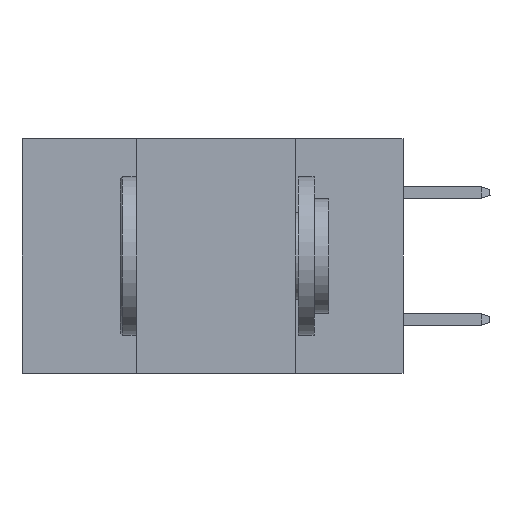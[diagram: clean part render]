
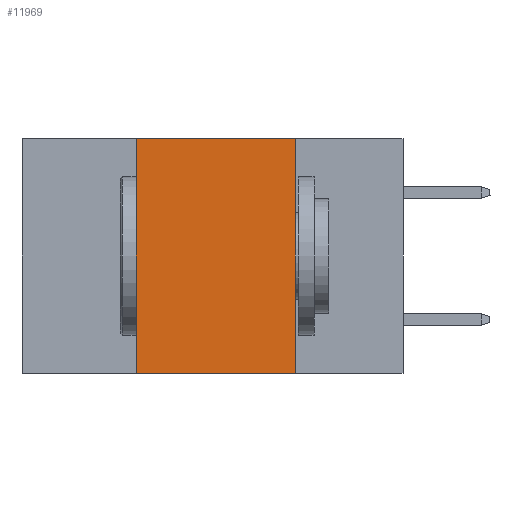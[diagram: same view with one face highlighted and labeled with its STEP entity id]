
A CAD part, left-side view. The second image highlights one B-rep face of the part: STEP entity #11969.
In plain terms, the highlighted planar face has unit normal (-1, 0, 0).
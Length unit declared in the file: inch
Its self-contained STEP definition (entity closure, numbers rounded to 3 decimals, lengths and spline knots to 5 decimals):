
#2005 = DIRECTION ( 'NONE',  ( 0., -1., 0. ) ) ;
#2212 = CARTESIAN_POINT ( 'NONE',  ( 0., 0.17, 0. ) ) ;
#2216 = EDGE_CURVE ( 'NONE', #22593, #23762, #4765, .T. ) ;
#3270 = CARTESIAN_POINT ( 'NONE',  ( 0., 0.42, -0.37 ) ) ;
#3376 = DIRECTION ( 'NONE',  ( 1., 0., 0. ) ) ;
#3824 = PLANE ( 'NONE',  #24201 ) ;
#3986 = VECTOR ( 'NONE', #5629, 39.37008 ) ;
#4765 = LINE ( 'NONE', #2212, #3986 ) ;
#5629 = DIRECTION ( 'NONE',  ( 0., 0., -1. ) ) ;
#5731 = ORIENTED_EDGE ( 'NONE', *, *, #12897, .T. ) ;
#11876 = VECTOR ( 'NONE', #23949, 39.37008 ) ;
#11969 = ADVANCED_FACE ( 'NONE', ( #19622 ), #3824, .F. ) ;
#12359 = LINE ( 'NONE', #41509, #41245 ) ;
#12588 = VECTOR ( 'NONE', #2005, 39.37008 ) ;
#12897 = EDGE_CURVE ( 'NONE', #41001, #23762, #27616, .T. ) ;
#13664 = CARTESIAN_POINT ( 'NONE',  ( 0., 0.17, 0. ) ) ;
#13856 = ORIENTED_EDGE ( 'NONE', *, *, #27637, .F. ) ;
#16826 = DIRECTION ( 'NONE',  ( 0., 0., -1. ) ) ;
#18151 = EDGE_CURVE ( 'NONE', #18789, #22593, #29124, .T. ) ;
#18230 = CARTESIAN_POINT ( 'NONE',  ( 0., 0.6, 0. ) ) ;
#18789 = VERTEX_POINT ( 'NONE', #37181 ) ;
#19622 = FACE_OUTER_BOUND ( 'NONE', #40034, .T. ) ;
#22593 = VERTEX_POINT ( 'NONE', #13664 ) ;
#23762 = VERTEX_POINT ( 'NONE', #29967 ) ;
#23949 = DIRECTION ( 'NONE',  ( 0., -1., 0. ) ) ;
#24201 = AXIS2_PLACEMENT_3D ( 'NONE', #39382, #3376, #16826 ) ;
#27616 = LINE ( 'NONE', #31256, #11876 ) ;
#27637 = EDGE_CURVE ( 'NONE', #41001, #18789, #12359, .T. ) ;
#29124 = LINE ( 'NONE', #18230, #12588 ) ;
#29967 = CARTESIAN_POINT ( 'NONE',  ( 0., 0.17, -0.37 ) ) ;
#31234 = DIRECTION ( 'NONE',  ( 0., 0., 1. ) ) ;
#31256 = CARTESIAN_POINT ( 'NONE',  ( 0., 0.6, -0.37 ) ) ;
#32502 = ORIENTED_EDGE ( 'NONE', *, *, #2216, .F. ) ;
#33096 = ORIENTED_EDGE ( 'NONE', *, *, #18151, .F. ) ;
#37181 = CARTESIAN_POINT ( 'NONE',  ( 0., 0.42, 0. ) ) ;
#39382 = CARTESIAN_POINT ( 'NONE',  ( 0., 0.6, 0. ) ) ;
#40034 = EDGE_LOOP ( 'NONE', ( #32502, #33096, #13856, #5731 ) ) ;
#41001 = VERTEX_POINT ( 'NONE', #3270 ) ;
#41245 = VECTOR ( 'NONE', #31234, 39.37008 ) ;
#41509 = CARTESIAN_POINT ( 'NONE',  ( 0., 0.42, 0. ) ) ;
